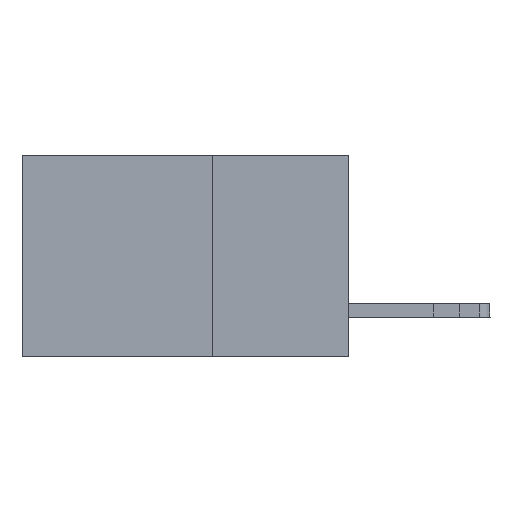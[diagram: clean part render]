
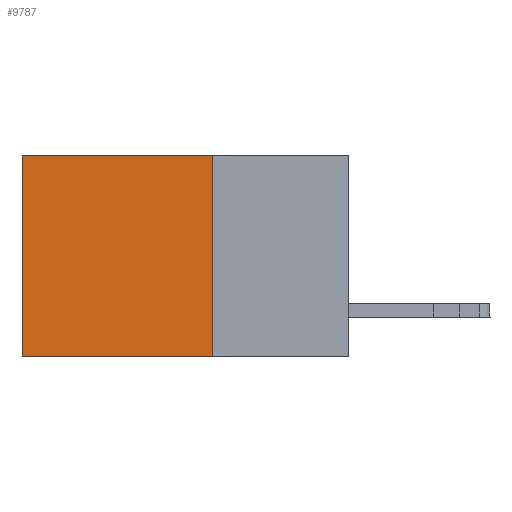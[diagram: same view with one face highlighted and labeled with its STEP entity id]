
A CAD part, left-side view. The second image highlights one B-rep face of the part: STEP entity #9787.
In plain terms, the highlighted planar face has unit normal (-1, 0, 0).
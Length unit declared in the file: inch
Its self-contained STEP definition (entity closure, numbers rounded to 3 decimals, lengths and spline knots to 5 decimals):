
#1715 = CARTESIAN_POINT ( 'NONE',  ( 0.298, 0.6, 0. ) ) ;
#1975 = ORIENTED_EDGE ( 'NONE', *, *, #11397, .F. ) ;
#3026 = CARTESIAN_POINT ( 'NONE',  ( 0.298, 0.25, -0.37 ) ) ;
#3589 = LINE ( 'NONE', #19141, #24105 ) ;
#3632 = ORIENTED_EDGE ( 'NONE', *, *, #23844, .T. ) ;
#4706 = FACE_OUTER_BOUND ( 'NONE', #8312, .T. ) ;
#4986 = LINE ( 'NONE', #9261, #7257 ) ;
#6116 = ORIENTED_EDGE ( 'NONE', *, *, #18405, .T. ) ;
#6751 = CARTESIAN_POINT ( 'NONE',  ( 0.298, 0.25, 0. ) ) ;
#7257 = VECTOR ( 'NONE', #18734, 39.37008 ) ;
#8312 = EDGE_LOOP ( 'NONE', ( #6116, #1975, #13047, #3632 ) ) ;
#9261 = CARTESIAN_POINT ( 'NONE',  ( 0.298, 0.6, 0. ) ) ;
#9787 = ADVANCED_FACE ( 'NONE', ( #4706 ), #10522, .F. ) ;
#9907 = AXIS2_PLACEMENT_3D ( 'NONE', #6751, #18458, #18699 ) ;
#10373 = CARTESIAN_POINT ( 'NONE',  ( 0.298, 0.6, -0.37 ) ) ;
#10505 = LINE ( 'NONE', #16094, #10946 ) ;
#10522 = PLANE ( 'NONE',  #9907 ) ;
#10946 = VECTOR ( 'NONE', #22318, 39.37008 ) ;
#11397 = EDGE_CURVE ( 'NONE', #21249, #21550, #20028, .T. ) ;
#11850 = VERTEX_POINT ( 'NONE', #20216 ) ;
#11973 = CARTESIAN_POINT ( 'NONE',  ( 0.298, 0.25, -0.37 ) ) ;
#12346 = VERTEX_POINT ( 'NONE', #1715 ) ;
#13047 = ORIENTED_EDGE ( 'NONE', *, *, #15107, .F. ) ;
#15107 = EDGE_CURVE ( 'NONE', #11850, #21249, #10505, .T. ) ;
#16094 = CARTESIAN_POINT ( 'NONE',  ( 0.298, 0.25, 0. ) ) ;
#17592 = DIRECTION ( 'NONE',  ( 0., 1., 0. ) ) ;
#18336 = DIRECTION ( 'NONE',  ( 0., 1., 0. ) ) ;
#18405 = EDGE_CURVE ( 'NONE', #12346, #21550, #4986, .T. ) ;
#18458 = DIRECTION ( 'NONE',  ( 1., 0., 0. ) ) ;
#18699 = DIRECTION ( 'NONE',  ( 0., 0., -1. ) ) ;
#18734 = DIRECTION ( 'NONE',  ( 0., 0., -1. ) ) ;
#19141 = CARTESIAN_POINT ( 'NONE',  ( 0.298, 0.25, 0. ) ) ;
#20028 = LINE ( 'NONE', #11973, #23664 ) ;
#20216 = CARTESIAN_POINT ( 'NONE',  ( 0.298, 0.25, 0. ) ) ;
#21249 = VERTEX_POINT ( 'NONE', #3026 ) ;
#21550 = VERTEX_POINT ( 'NONE', #10373 ) ;
#22318 = DIRECTION ( 'NONE',  ( 0., 0., -1. ) ) ;
#23664 = VECTOR ( 'NONE', #18336, 39.37008 ) ;
#23844 = EDGE_CURVE ( 'NONE', #11850, #12346, #3589, .T. ) ;
#24105 = VECTOR ( 'NONE', #17592, 39.37008 ) ;
